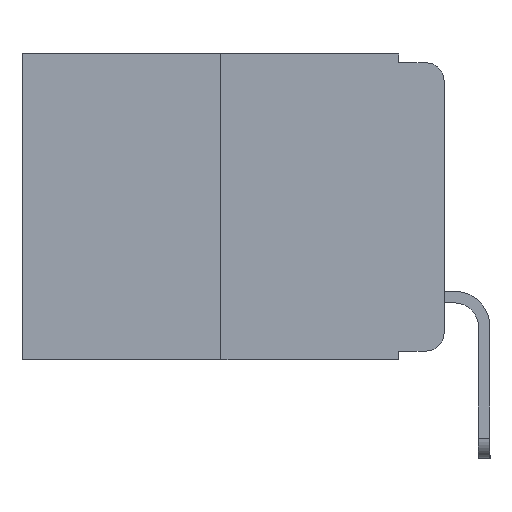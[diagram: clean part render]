
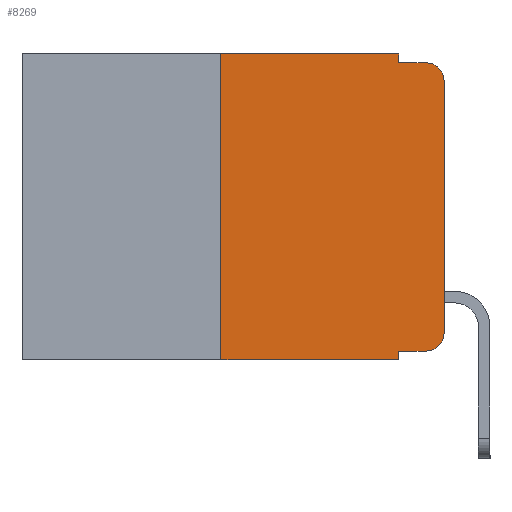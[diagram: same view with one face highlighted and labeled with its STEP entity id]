
A CAD part, left-side view. The second image highlights one B-rep face of the part: STEP entity #8269.
In plain terms, the highlighted planar face has unit normal (-1, 0, 0).
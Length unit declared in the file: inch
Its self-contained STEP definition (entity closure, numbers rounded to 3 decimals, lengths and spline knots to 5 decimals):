
#10 = CARTESIAN_POINT ( 'NONE',  ( 0., 0.051, -0.01 ) ) ;
#188 = ORIENTED_EDGE ( 'NONE', *, *, #6808, .T. ) ;
#356 = VECTOR ( 'NONE', #10916, 39.37008 ) ;
#423 = EDGE_CURVE ( 'NONE', #5142, #1330, #9838, .T. ) ;
#459 = AXIS2_PLACEMENT_3D ( 'NONE', #3156, #905, #4195 ) ;
#593 = VERTEX_POINT ( 'NONE', #9105 ) ;
#687 = CIRCLE ( 'NONE', #459, 0.02 ) ;
#688 = CARTESIAN_POINT ( 'NONE',  ( 0., 0.051, -0.333 ) ) ;
#718 = LINE ( 'NONE', #8049, #10870 ) ;
#745 = EDGE_CURVE ( 'NONE', #11135, #6882, #2005, .T. ) ;
#865 = LINE ( 'NONE', #6457, #9114 ) ;
#905 = DIRECTION ( 'NONE',  ( -1., 0., 0. ) ) ;
#1210 = DIRECTION ( 'NONE',  ( 0., -1., 0. ) ) ;
#1287 = CARTESIAN_POINT ( 'NONE',  ( 0., 0.051, 0. ) ) ;
#1330 = VERTEX_POINT ( 'NONE', #9714 ) ;
#1381 = EDGE_CURVE ( 'NONE', #11774, #9813, #6639, .T. ) ;
#1419 = CARTESIAN_POINT ( 'NONE',  ( 0., 0.051, 0. ) ) ;
#1621 = VECTOR ( 'NONE', #13070, 39.37008 ) ;
#1628 = ORIENTED_EDGE ( 'NONE', *, *, #1381, .T. ) ;
#2005 = LINE ( 'NONE', #13706, #11186 ) ;
#2027 = ORIENTED_EDGE ( 'NONE', *, *, #423, .F. ) ;
#2227 = VERTEX_POINT ( 'NONE', #1287 ) ;
#2645 = ORIENTED_EDGE ( 'NONE', *, *, #12471, .T. ) ;
#2737 = CARTESIAN_POINT ( 'NONE',  ( 0., 0., -0.03 ) ) ;
#3122 = DIRECTION ( 'NONE',  ( 0., 0., 1. ) ) ;
#3156 = CARTESIAN_POINT ( 'NONE',  ( 0., 0.02, -0.03 ) ) ;
#3176 = CARTESIAN_POINT ( 'NONE',  ( 0., 0.473, -0.343 ) ) ;
#3261 = EDGE_LOOP ( 'NONE', ( #1628, #2645, #2027, #4078, #10328, #8314, #12789, #8936, #11045, #188 ) ) ;
#3568 = CARTESIAN_POINT ( 'NONE',  ( 0., 0., 0. ) ) ;
#3634 = CARTESIAN_POINT ( 'NONE',  ( 0., 0.051, -0.01 ) ) ;
#3852 = EDGE_CURVE ( 'NONE', #11135, #5953, #12671, .T. ) ;
#4078 = ORIENTED_EDGE ( 'NONE', *, *, #5804, .F. ) ;
#4195 = DIRECTION ( 'NONE',  ( 0., 0., -1. ) ) ;
#4407 = DIRECTION ( 'NONE',  ( 0., 0., 1. ) ) ;
#4447 = FACE_OUTER_BOUND ( 'NONE', #3261, .T. ) ;
#4786 = CARTESIAN_POINT ( 'NONE',  ( 0., 0.051, 0. ) ) ;
#5142 = VERTEX_POINT ( 'NONE', #3634 ) ;
#5367 = VERTEX_POINT ( 'NONE', #688 ) ;
#5420 = LINE ( 'NONE', #1419, #356 ) ;
#5804 = EDGE_CURVE ( 'NONE', #2227, #5142, #5420, .T. ) ;
#5851 = VECTOR ( 'NONE', #1210, 39.37008 ) ;
#5953 = VERTEX_POINT ( 'NONE', #11048 ) ;
#6457 = CARTESIAN_POINT ( 'NONE',  ( 0., 0.051, -0.333 ) ) ;
#6473 = DIRECTION ( 'NONE',  ( 1., 0., 0. ) ) ;
#6639 = LINE ( 'NONE', #3568, #12091 ) ;
#6808 = EDGE_CURVE ( 'NONE', #593, #11774, #11755, .T. ) ;
#6827 = AXIS2_PLACEMENT_3D ( 'NONE', #7867, #11148, #6879 ) ;
#6836 = CARTESIAN_POINT ( 'NONE',  ( 0., 0.25, -0.343 ) ) ;
#6879 = DIRECTION ( 'NONE',  ( 0., 0., -1. ) ) ;
#6882 = VERTEX_POINT ( 'NONE', #6950 ) ;
#6950 = CARTESIAN_POINT ( 'NONE',  ( 0., 0.25, 0. ) ) ;
#7645 = CARTESIAN_POINT ( 'NONE',  ( 0., 0.473, 0. ) ) ;
#7802 = VECTOR ( 'NONE', #9034, 39.37008 ) ;
#7867 = CARTESIAN_POINT ( 'NONE',  ( 0., 0.02, -0.313 ) ) ;
#8049 = CARTESIAN_POINT ( 'NONE',  ( 0., 0.473, 0. ) ) ;
#8269 = ADVANCED_FACE ( 'NONE', ( #4447 ), #12986, .F. ) ;
#8314 = ORIENTED_EDGE ( 'NONE', *, *, #745, .F. ) ;
#8936 = ORIENTED_EDGE ( 'NONE', *, *, #11934, .F. ) ;
#9033 = EDGE_CURVE ( 'NONE', #6882, #2227, #718, .T. ) ;
#9034 = DIRECTION ( 'NONE',  ( 0., 0., -1. ) ) ;
#9105 = CARTESIAN_POINT ( 'NONE',  ( 0., 0.02, -0.333 ) ) ;
#9114 = VECTOR ( 'NONE', #11551, 39.37008 ) ;
#9714 = CARTESIAN_POINT ( 'NONE',  ( 0., 0.02, -0.01 ) ) ;
#9813 = VERTEX_POINT ( 'NONE', #2737 ) ;
#9838 = LINE ( 'NONE', #10, #1621 ) ;
#10017 = LINE ( 'NONE', #4786, #7802 ) ;
#10328 = ORIENTED_EDGE ( 'NONE', *, *, #9033, .F. ) ;
#10399 = EDGE_CURVE ( 'NONE', #5367, #593, #865, .T. ) ;
#10870 = VECTOR ( 'NONE', #13674, 39.37008 ) ;
#10916 = DIRECTION ( 'NONE',  ( 0., 0., -1. ) ) ;
#11045 = ORIENTED_EDGE ( 'NONE', *, *, #10399, .T. ) ;
#11048 = CARTESIAN_POINT ( 'NONE',  ( 0., 0.051, -0.343 ) ) ;
#11135 = VERTEX_POINT ( 'NONE', #6836 ) ;
#11148 = DIRECTION ( 'NONE',  ( -1., 0., 0. ) ) ;
#11186 = VECTOR ( 'NONE', #3122, 39.37008 ) ;
#11551 = DIRECTION ( 'NONE',  ( 0., -1., 0. ) ) ;
#11755 = CIRCLE ( 'NONE', #6827, 0.02 ) ;
#11774 = VERTEX_POINT ( 'NONE', #11869 ) ;
#11789 = DIRECTION ( 'NONE',  ( 0., 0., -1. ) ) ;
#11869 = CARTESIAN_POINT ( 'NONE',  ( 0., 0., -0.313 ) ) ;
#11934 = EDGE_CURVE ( 'NONE', #5367, #5953, #10017, .T. ) ;
#12091 = VECTOR ( 'NONE', #4407, 39.37008 ) ;
#12455 = AXIS2_PLACEMENT_3D ( 'NONE', #7645, #6473, #11789 ) ;
#12471 = EDGE_CURVE ( 'NONE', #9813, #1330, #687, .T. ) ;
#12671 = LINE ( 'NONE', #3176, #5851 ) ;
#12789 = ORIENTED_EDGE ( 'NONE', *, *, #3852, .T. ) ;
#12986 = PLANE ( 'NONE',  #12455 ) ;
#13070 = DIRECTION ( 'NONE',  ( 0., -1., 0. ) ) ;
#13674 = DIRECTION ( 'NONE',  ( 0., -1., 0. ) ) ;
#13706 = CARTESIAN_POINT ( 'NONE',  ( 0., 0.25, 0. ) ) ;
